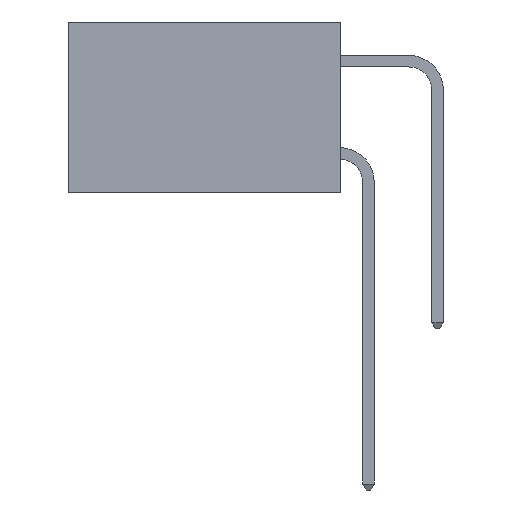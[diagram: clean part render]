
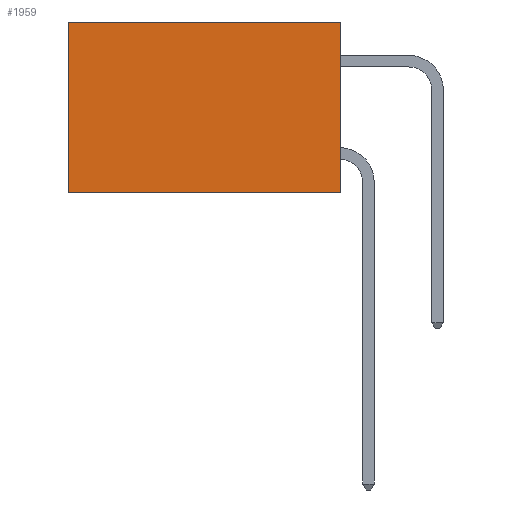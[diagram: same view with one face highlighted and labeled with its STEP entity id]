
A CAD part, left-side view. The second image highlights one B-rep face of the part: STEP entity #1959.
In plain terms, the highlighted planar face has unit normal (-1, 0, 0).
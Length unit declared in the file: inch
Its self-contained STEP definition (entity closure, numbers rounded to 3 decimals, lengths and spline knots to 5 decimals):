
#29 = CARTESIAN_POINT ( 'NONE',  ( 0.277, 0., -0.37 ) ) ;
#310 = FACE_OUTER_BOUND ( 'NONE', #5845, .T. ) ;
#538 = PLANE ( 'NONE',  #1941 ) ;
#559 = CARTESIAN_POINT ( 'NONE',  ( 0.277, 0., -0.37 ) ) ;
#789 = DIRECTION ( 'NONE',  ( 0., 1., 0. ) ) ;
#845 = ORIENTED_EDGE ( 'NONE', *, *, #5004, .T. ) ;
#1263 = DIRECTION ( 'NONE',  ( 1., 0., 0. ) ) ;
#1279 = ORIENTED_EDGE ( 'NONE', *, *, #2223, .F. ) ;
#1495 = ORIENTED_EDGE ( 'NONE', *, *, #2642, .F. ) ;
#1726 = EDGE_CURVE ( 'NONE', #2075, #3913, #7932, .T. ) ;
#1941 = AXIS2_PLACEMENT_3D ( 'NONE', #3458, #1263, #6381 ) ;
#1959 = ADVANCED_FACE ( 'NONE', ( #310 ), #538, .F. ) ;
#2075 = VERTEX_POINT ( 'NONE', #8630 ) ;
#2136 = CARTESIAN_POINT ( 'NONE',  ( 0.277, 0., -0.37 ) ) ;
#2223 = EDGE_CURVE ( 'NONE', #5268, #8198, #5807, .T. ) ;
#2359 = VECTOR ( 'NONE', #9226, 39.37008 ) ;
#2642 = EDGE_CURVE ( 'NONE', #2075, #5268, #8373, .T. ) ;
#2811 = ORIENTED_EDGE ( 'NONE', *, *, #1726, .T. ) ;
#3458 = CARTESIAN_POINT ( 'NONE',  ( 0.277, 0., -0.37 ) ) ;
#3909 = DIRECTION ( 'NONE',  ( 0., 1., 0. ) ) ;
#3913 = VERTEX_POINT ( 'NONE', #4318 ) ;
#4075 = CARTESIAN_POINT ( 'NONE',  ( 0.277, 0.59, -0.37 ) ) ;
#4318 = CARTESIAN_POINT ( 'NONE',  ( 0.277, 0.59, 0. ) ) ;
#5004 = EDGE_CURVE ( 'NONE', #3913, #8198, #5641, .T. ) ;
#5268 = VERTEX_POINT ( 'NONE', #2136 ) ;
#5534 = CARTESIAN_POINT ( 'NONE',  ( 0.277, 0.59, -0.37 ) ) ;
#5641 = LINE ( 'NONE', #5534, #9218 ) ;
#5807 = LINE ( 'NONE', #29, #9358 ) ;
#5845 = EDGE_LOOP ( 'NONE', ( #845, #1279, #1495, #2811 ) ) ;
#6266 = DIRECTION ( 'NONE',  ( 0., 0., -1. ) ) ;
#6381 = DIRECTION ( 'NONE',  ( 0., 0., -1. ) ) ;
#7932 = LINE ( 'NONE', #8230, #8170 ) ;
#8170 = VECTOR ( 'NONE', #3909, 39.37008 ) ;
#8198 = VERTEX_POINT ( 'NONE', #4075 ) ;
#8230 = CARTESIAN_POINT ( 'NONE',  ( 0.277, 0., 0. ) ) ;
#8373 = LINE ( 'NONE', #559, #2359 ) ;
#8630 = CARTESIAN_POINT ( 'NONE',  ( 0.277, 0., 0. ) ) ;
#9218 = VECTOR ( 'NONE', #6266, 39.37008 ) ;
#9226 = DIRECTION ( 'NONE',  ( 0., 0., -1. ) ) ;
#9358 = VECTOR ( 'NONE', #789, 39.37008 ) ;
